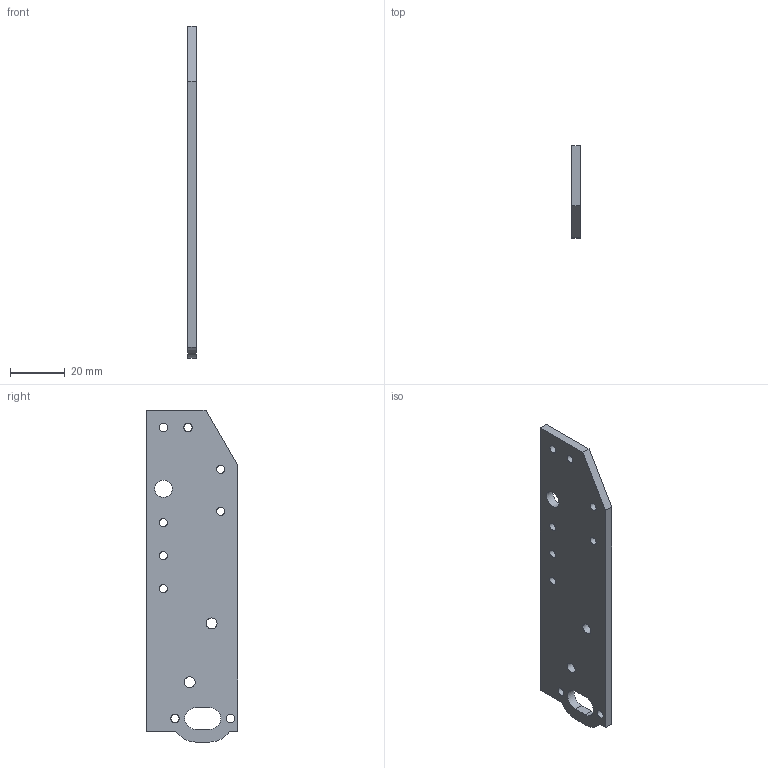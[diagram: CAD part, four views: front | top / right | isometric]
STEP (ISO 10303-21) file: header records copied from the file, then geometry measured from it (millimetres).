
FILE_DESCRIPTION (( 'STEP AP214' ), '1' );
FILE_NAME ('No_Safety_Reinforced_Side_Right.step', '2016-01-30T20:06:15', ( 'WarFairy' ), ( '' ), 'SwSTEP 2.0', 'SolidWorks 2015', '' );
FILE_SCHEMA (( 'AUTOMOTIVE_DESIGN' ));
Length unit declared in the file: millimetre
Products named in the file (1): No_Safety_Reinforced_Side_Right
Bounding box: 3.17 x 33.43 x 120.78 mm (x, y, z)
Volume: 11528.8 mm3; surface area: 8747.8 mm2
Topology: 1 solids, 1 shells, 41 faces, 111 edges, 74 vertices
Faces by surface type: plane 25, cylinder 16
Full cylindrical faces by diameter (mm): 3 x9, 3.97 x2, 6.35 x1
Entity records: 1323 total; most frequent: CARTESIAN_POINT 215, DIRECTION 215, ORIENTED_EDGE 198, EDGE_CURVE 99, EDGE_LOOP 81, AXIS2_PLACEMENT_3D 74, VERTEX_POINT 74, VECTOR 67
